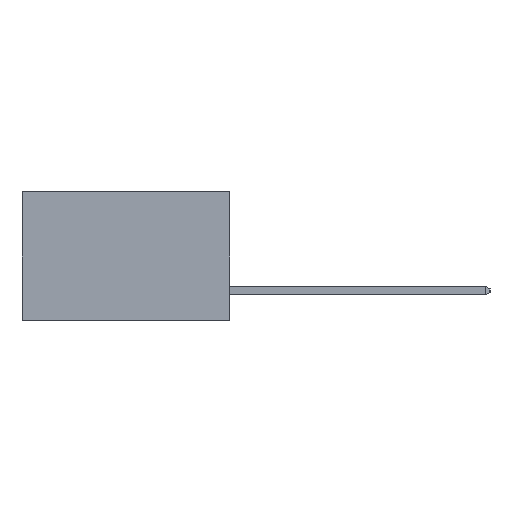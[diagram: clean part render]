
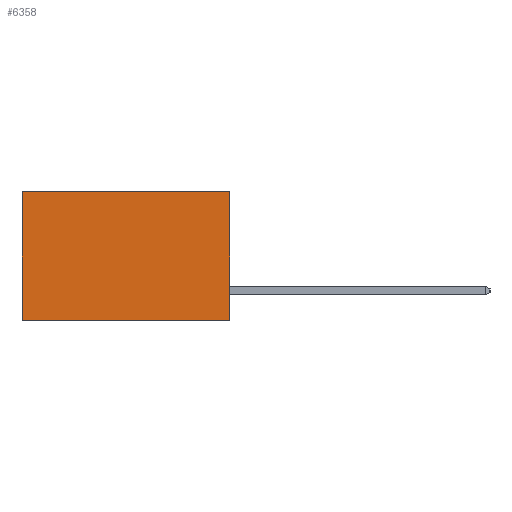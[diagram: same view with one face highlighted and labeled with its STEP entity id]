
A CAD part, left-side view. The second image highlights one B-rep face of the part: STEP entity #6358.
In plain terms, the highlighted planar face has unit normal (-1, 0, 0).
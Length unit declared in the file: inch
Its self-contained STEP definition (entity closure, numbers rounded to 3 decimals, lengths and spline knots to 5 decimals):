
#808 = LINE ( 'NONE', #7630, #5789 ) ;
#1000 = DIRECTION ( 'NONE',  ( 0., 0., -1. ) ) ;
#1208 = ORIENTED_EDGE ( 'NONE', *, *, #1642, .F. ) ;
#1240 = EDGE_LOOP ( 'NONE', ( #12204, #8048, #1208, #4024 ) ) ;
#1469 = LINE ( 'NONE', #5833, #6428 ) ;
#1642 = EDGE_CURVE ( 'NONE', #7242, #4217, #12858, .T. ) ;
#2160 = CARTESIAN_POINT ( 'NONE',  ( 0.2615, 0., 0. ) ) ;
#2398 = DIRECTION ( 'NONE',  ( 0., 1., 0. ) ) ;
#3524 = CARTESIAN_POINT ( 'NONE',  ( 0.2615, 0., -0.37 ) ) ;
#4024 = ORIENTED_EDGE ( 'NONE', *, *, #9069, .T. ) ;
#4217 = VERTEX_POINT ( 'NONE', #3524 ) ;
#4631 = EDGE_CURVE ( 'NONE', #6294, #6314, #808, .T. ) ;
#5050 = AXIS2_PLACEMENT_3D ( 'NONE', #12006, #11940, #11919 ) ;
#5540 = CARTESIAN_POINT ( 'NONE',  ( 0.2615, 0., -0.37 ) ) ;
#5789 = VECTOR ( 'NONE', #11718, 39.37008 ) ;
#5790 = EDGE_CURVE ( 'NONE', #4217, #6314, #12898, .T. ) ;
#5833 = CARTESIAN_POINT ( 'NONE',  ( 0.2615, 0., 0. ) ) ;
#6294 = VERTEX_POINT ( 'NONE', #12666 ) ;
#6314 = VERTEX_POINT ( 'NONE', #12407 ) ;
#6358 = ADVANCED_FACE ( 'NONE', ( #12714 ), #12048, .F. ) ;
#6428 = VECTOR ( 'NONE', #6819, 39.37008 ) ;
#6819 = DIRECTION ( 'NONE',  ( 0., 1., 0. ) ) ;
#7242 = VERTEX_POINT ( 'NONE', #2160 ) ;
#7630 = CARTESIAN_POINT ( 'NONE',  ( 0.2615, 0.6, -0.37 ) ) ;
#7794 = CARTESIAN_POINT ( 'NONE',  ( 0.2615, 0., -0.37 ) ) ;
#8048 = ORIENTED_EDGE ( 'NONE', *, *, #5790, .F. ) ;
#9069 = EDGE_CURVE ( 'NONE', #7242, #6294, #1469, .T. ) ;
#10276 = VECTOR ( 'NONE', #1000, 39.37008 ) ;
#10310 = VECTOR ( 'NONE', #2398, 39.37008 ) ;
#11718 = DIRECTION ( 'NONE',  ( 0., 0., -1. ) ) ;
#11919 = DIRECTION ( 'NONE',  ( 0., 0., -1. ) ) ;
#11940 = DIRECTION ( 'NONE',  ( 1., 0., 0. ) ) ;
#12006 = CARTESIAN_POINT ( 'NONE',  ( 0.2615, 0., -0.37 ) ) ;
#12048 = PLANE ( 'NONE',  #5050 ) ;
#12204 = ORIENTED_EDGE ( 'NONE', *, *, #4631, .T. ) ;
#12407 = CARTESIAN_POINT ( 'NONE',  ( 0.2615, 0.6, -0.37 ) ) ;
#12666 = CARTESIAN_POINT ( 'NONE',  ( 0.2615, 0.6, 0. ) ) ;
#12714 = FACE_OUTER_BOUND ( 'NONE', #1240, .T. ) ;
#12858 = LINE ( 'NONE', #5540, #10276 ) ;
#12898 = LINE ( 'NONE', #7794, #10310 ) ;
